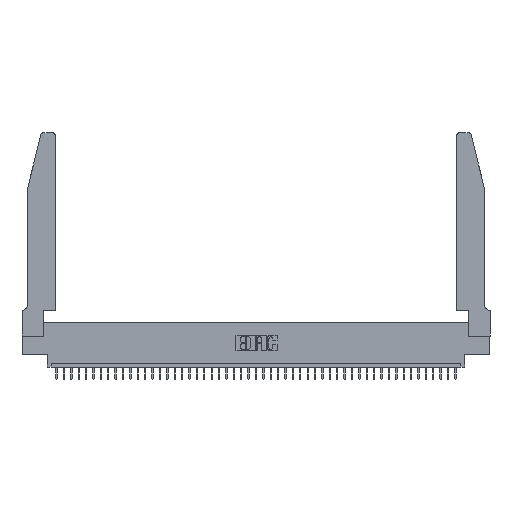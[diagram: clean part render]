
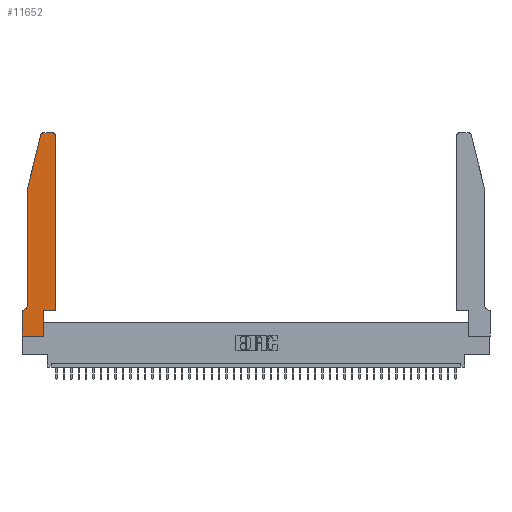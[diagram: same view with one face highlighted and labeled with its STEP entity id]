
A CAD part, top view. The second image highlights one B-rep face of the part: STEP entity #11652.
In plain terms, the highlighted planar face has unit normal (0, 0, 1).
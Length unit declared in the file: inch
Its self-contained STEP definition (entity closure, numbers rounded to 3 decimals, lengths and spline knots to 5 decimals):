
#827 = CARTESIAN_POINT ( 'NONE',  ( 0.0755, 2., 0.37 ) ) ;
#2774 = DIRECTION ( 'NONE',  ( -1., 0., 0. ) ) ;
#2998 = EDGE_CURVE ( 'NONE', #34495, #40132, #5943, .T. ) ;
#3106 = DIRECTION ( 'NONE',  ( 0., 1., 0. ) ) ;
#3735 = CARTESIAN_POINT ( 'NONE',  ( 0., 0., 0.37 ) ) ;
#3745 = ORIENTED_EDGE ( 'NONE', *, *, #12813, .T. ) ;
#4154 = CARTESIAN_POINT ( 'NONE',  ( 0.0055, 0.35, 0.37 ) ) ;
#4922 = CIRCLE ( 'NONE', #8736, 0.03 ) ;
#5646 = CIRCLE ( 'NONE', #36948, 0.07 ) ;
#5943 = LINE ( 'NONE', #18499, #39315 ) ;
#6431 = AXIS2_PLACEMENT_3D ( 'NONE', #28828, #42027, #28680 ) ;
#6446 = ORIENTED_EDGE ( 'NONE', *, *, #28969, .T. ) ;
#6640 = EDGE_CURVE ( 'NONE', #40336, #8179, #41516, .T. ) ;
#7620 = DIRECTION ( 'NONE',  ( 1., 0., 0. ) ) ;
#7975 = ORIENTED_EDGE ( 'NONE', *, *, #37571, .T. ) ;
#8179 = VERTEX_POINT ( 'NONE', #16581 ) ;
#8736 = AXIS2_PLACEMENT_3D ( 'NONE', #14120, #27695, #20899 ) ;
#9115 = VERTEX_POINT ( 'NONE', #30789 ) ;
#9303 = VECTOR ( 'NONE', #27981, 39.37008 ) ;
#10406 = CIRCLE ( 'NONE', #25412, 0.03 ) ;
#10939 = EDGE_CURVE ( 'NONE', #13425, #30631, #5646, .T. ) ;
#11106 = DIRECTION ( 'NONE',  ( -0.239, -0.971, 0. ) ) ;
#11445 = VERTEX_POINT ( 'NONE', #11531 ) ;
#11531 = CARTESIAN_POINT ( 'NONE',  ( 0., 0., 0.37 ) ) ;
#11652 = ADVANCED_FACE ( 'NONE', ( #29605 ), #15111, .T. ) ;
#11656 = ORIENTED_EDGE ( 'NONE', *, *, #24752, .T. ) ;
#12213 = VECTOR ( 'NONE', #44268, 39.37008 ) ;
#12262 = ORIENTED_EDGE ( 'NONE', *, *, #34149, .T. ) ;
#12813 = EDGE_CURVE ( 'NONE', #43092, #13425, #37578, .T. ) ;
#13300 = CARTESIAN_POINT ( 'NONE',  ( 0.0755, 2., 0.37 ) ) ;
#13425 = VERTEX_POINT ( 'NONE', #43132 ) ;
#14120 = CARTESIAN_POINT ( 'NONE',  ( 0.284, 2.72, 0.37 ) ) ;
#15111 = PLANE ( 'NONE',  #6431 ) ;
#15225 = EDGE_CURVE ( 'NONE', #25951, #11445, #31898, .T. ) ;
#16553 = DIRECTION ( 'NONE',  ( 0., 1., 0. ) ) ;
#16581 = CARTESIAN_POINT ( 'NONE',  ( 0.284, 2.75, 0.37 ) ) ;
#16664 = VECTOR ( 'NONE', #16553, 39.37008 ) ;
#16783 = ORIENTED_EDGE ( 'NONE', *, *, #44023, .T. ) ;
#16830 = VECTOR ( 'NONE', #21456, 39.37008 ) ;
#17935 = LINE ( 'NONE', #827, #30337 ) ;
#18499 = CARTESIAN_POINT ( 'NONE',  ( 0.4505, 0.35, 0.37 ) ) ;
#20899 = DIRECTION ( 'NONE',  ( 1., 0., 0. ) ) ;
#20995 = LINE ( 'NONE', #40994, #42500 ) ;
#21456 = DIRECTION ( 'NONE',  ( -1., 0., 0. ) ) ;
#21795 = CARTESIAN_POINT ( 'NONE',  ( 0.2865, 0.35, 0.37 ) ) ;
#22242 = VECTOR ( 'NONE', #3106, 39.37008 ) ;
#22291 = CARTESIAN_POINT ( 'NONE',  ( 0.2605, 2.75, 0.37 ) ) ;
#23782 = CARTESIAN_POINT ( 'NONE',  ( 0.0055, 0.42, 0.37 ) ) ;
#24174 = LINE ( 'NONE', #37163, #16664 ) ;
#24644 = DIRECTION ( 'NONE',  ( -1., 0., 0. ) ) ;
#24752 = EDGE_CURVE ( 'NONE', #30631, #25951, #20995, .T. ) ;
#25412 = AXIS2_PLACEMENT_3D ( 'NONE', #35622, #39091, #43447 ) ;
#25652 = CARTESIAN_POINT ( 'NONE',  ( 0.4205, 2.75, 0.37 ) ) ;
#25760 = LINE ( 'NONE', #44328, #22242 ) ;
#25951 = VERTEX_POINT ( 'NONE', #26421 ) ;
#26421 = CARTESIAN_POINT ( 'NONE',  ( 0., 0.35, 0.37 ) ) ;
#27695 = DIRECTION ( 'NONE',  ( 0., 0., 1. ) ) ;
#27798 = CARTESIAN_POINT ( 'NONE',  ( 0.25487, 2.72718, 0.37 ) ) ;
#27981 = DIRECTION ( 'NONE',  ( 0., -1., 0. ) ) ;
#28680 = DIRECTION ( 'NONE',  ( 1., 0., 0. ) ) ;
#28828 = CARTESIAN_POINT ( 'NONE',  ( 0., 0.35, 0.37 ) ) ;
#28969 = EDGE_CURVE ( 'NONE', #9115, #40336, #10406, .T. ) ;
#29605 = FACE_OUTER_BOUND ( 'NONE', #34006, .T. ) ;
#30337 = VECTOR ( 'NONE', #11106, 39.37008 ) ;
#30631 = VERTEX_POINT ( 'NONE', #4154 ) ;
#30663 = DIRECTION ( 'NONE',  ( 1., 0., 0. ) ) ;
#30789 = CARTESIAN_POINT ( 'NONE',  ( 0.4505, 2.72, 0.37 ) ) ;
#31486 = CARTESIAN_POINT ( 'NONE',  ( 0.4505, 0.35, 0.37 ) ) ;
#31548 = ORIENTED_EDGE ( 'NONE', *, *, #10939, .T. ) ;
#31898 = LINE ( 'NONE', #3735, #9303 ) ;
#32449 = ORIENTED_EDGE ( 'NONE', *, *, #33978, .T. ) ;
#33171 = VECTOR ( 'NONE', #30663, 39.37008 ) ;
#33709 = ORIENTED_EDGE ( 'NONE', *, *, #2998, .T. ) ;
#33978 = EDGE_CURVE ( 'NONE', #40132, #9115, #25760, .T. ) ;
#34006 = EDGE_LOOP ( 'NONE', ( #44020, #34422, #16783, #3745, #31548, #11656, #40363, #7975, #12262, #33709, #32449, #6446 ) ) ;
#34149 = EDGE_CURVE ( 'NONE', #39041, #34495, #24174, .T. ) ;
#34275 = CARTESIAN_POINT ( 'NONE',  ( 0., 0., 0.37 ) ) ;
#34422 = ORIENTED_EDGE ( 'NONE', *, *, #44532, .T. ) ;
#34495 = VERTEX_POINT ( 'NONE', #21795 ) ;
#35622 = CARTESIAN_POINT ( 'NONE',  ( 0.4205, 2.72, 0.37 ) ) ;
#36423 = LINE ( 'NONE', #34275, #33171 ) ;
#36948 = AXIS2_PLACEMENT_3D ( 'NONE', #23782, #37624, #24644 ) ;
#36957 = CARTESIAN_POINT ( 'NONE',  ( 0.2865, 0., 0.37 ) ) ;
#37163 = CARTESIAN_POINT ( 'NONE',  ( 0.2865, 0.35, 0.37 ) ) ;
#37571 = EDGE_CURVE ( 'NONE', #11445, #39041, #36423, .T. ) ;
#37578 = LINE ( 'NONE', #13300, #12213 ) ;
#37624 = DIRECTION ( 'NONE',  ( 0., 0., -1. ) ) ;
#39041 = VERTEX_POINT ( 'NONE', #36957 ) ;
#39091 = DIRECTION ( 'NONE',  ( 0., 0., 1. ) ) ;
#39315 = VECTOR ( 'NONE', #7620, 39.37008 ) ;
#40132 = VERTEX_POINT ( 'NONE', #31486 ) ;
#40336 = VERTEX_POINT ( 'NONE', #25652 ) ;
#40363 = ORIENTED_EDGE ( 'NONE', *, *, #15225, .T. ) ;
#40868 = CARTESIAN_POINT ( 'NONE',  ( 0.0755, 2., 0.37 ) ) ;
#40994 = CARTESIAN_POINT ( 'NONE',  ( 0.0755, 0.35, 0.37 ) ) ;
#41516 = LINE ( 'NONE', #22291, #16830 ) ;
#42027 = DIRECTION ( 'NONE',  ( 0., 0., 1. ) ) ;
#42500 = VECTOR ( 'NONE', #2774, 39.37008 ) ;
#43092 = VERTEX_POINT ( 'NONE', #40868 ) ;
#43132 = CARTESIAN_POINT ( 'NONE',  ( 0.0755, 0.42, 0.37 ) ) ;
#43213 = VERTEX_POINT ( 'NONE', #27798 ) ;
#43447 = DIRECTION ( 'NONE',  ( 1., 0., 0. ) ) ;
#44020 = ORIENTED_EDGE ( 'NONE', *, *, #6640, .T. ) ;
#44023 = EDGE_CURVE ( 'NONE', #43213, #43092, #17935, .T. ) ;
#44268 = DIRECTION ( 'NONE',  ( 0., -1., 0. ) ) ;
#44328 = CARTESIAN_POINT ( 'NONE',  ( 0.4505, 0.35, 0.37 ) ) ;
#44532 = EDGE_CURVE ( 'NONE', #8179, #43213, #4922, .T. ) ;
